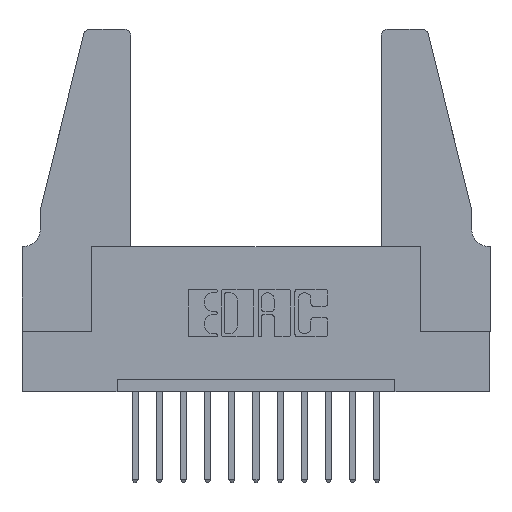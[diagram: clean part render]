
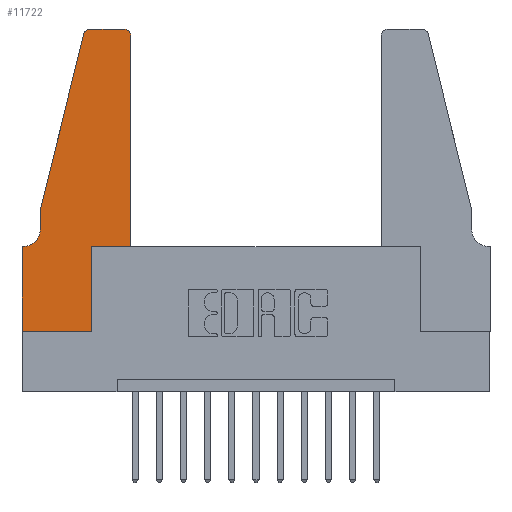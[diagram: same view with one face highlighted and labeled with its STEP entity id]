
A CAD part, top view. The second image highlights one B-rep face of the part: STEP entity #11722.
In plain terms, the highlighted planar face has unit normal (0, 0, 1).
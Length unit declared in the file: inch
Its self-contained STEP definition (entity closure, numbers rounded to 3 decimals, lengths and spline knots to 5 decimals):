
#106 = CARTESIAN_POINT ( 'NONE',  ( 0.2865, 0.35, 0.37 ) ) ;
#184 = VECTOR ( 'NONE', #12779, 39.37008 ) ;
#255 = DIRECTION ( 'NONE',  ( 1., 0., 0. ) ) ;
#328 = EDGE_CURVE ( 'NONE', #9432, #8564, #1690, .T. ) ;
#523 = EDGE_CURVE ( 'NONE', #2297, #10286, #2385, .T. ) ;
#626 = CARTESIAN_POINT ( 'NONE',  ( 0.2865, 0.35, 0.37 ) ) ;
#1080 = VECTOR ( 'NONE', #8777, 39.37008 ) ;
#1159 = VERTEX_POINT ( 'NONE', #5173 ) ;
#1486 = DIRECTION ( 'NONE',  ( 0., 1., 0. ) ) ;
#1690 = LINE ( 'NONE', #4432, #4351 ) ;
#1778 = DIRECTION ( 'NONE',  ( 0., 0., 1. ) ) ;
#2086 = FACE_OUTER_BOUND ( 'NONE', #7490, .T. ) ;
#2182 = AXIS2_PLACEMENT_3D ( 'NONE', #9927, #2772, #255 ) ;
#2297 = VERTEX_POINT ( 'NONE', #6164 ) ;
#2361 = DIRECTION ( 'NONE',  ( 1., 0., 0. ) ) ;
#2385 = LINE ( 'NONE', #5714, #5429 ) ;
#2461 = LINE ( 'NONE', #3813, #184 ) ;
#2501 = LINE ( 'NONE', #11528, #12940 ) ;
#2772 = DIRECTION ( 'NONE',  ( 0., 0., 1. ) ) ;
#2889 = EDGE_CURVE ( 'NONE', #3412, #6886, #9743, .T. ) ;
#2923 = PLANE ( 'NONE',  #6577 ) ;
#3412 = VERTEX_POINT ( 'NONE', #5383 ) ;
#3575 = DIRECTION ( 'NONE',  ( -1., 0., 0. ) ) ;
#3598 = VERTEX_POINT ( 'NONE', #626 ) ;
#3783 = ORIENTED_EDGE ( 'NONE', *, *, #9780, .T. ) ;
#3813 = CARTESIAN_POINT ( 'NONE',  ( 0., 0., 0.37 ) ) ;
#3838 = VERTEX_POINT ( 'NONE', #14155 ) ;
#4065 = VECTOR ( 'NONE', #5599, 39.37008 ) ;
#4280 = EDGE_CURVE ( 'NONE', #4663, #13851, #6752, .T. ) ;
#4351 = VECTOR ( 'NONE', #1486, 39.37008 ) ;
#4400 = ORIENTED_EDGE ( 'NONE', *, *, #328, .T. ) ;
#4432 = CARTESIAN_POINT ( 'NONE',  ( 0.4505, 0.35, 0.37 ) ) ;
#4453 = LINE ( 'NONE', #106, #7327 ) ;
#4565 = VECTOR ( 'NONE', #3575, 39.37008 ) ;
#4603 = CARTESIAN_POINT ( 'NONE',  ( 0.4205, 1.22, 0.37 ) ) ;
#4663 = VERTEX_POINT ( 'NONE', #6676 ) ;
#4938 = EDGE_CURVE ( 'NONE', #6886, #1159, #13020, .T. ) ;
#5011 = CARTESIAN_POINT ( 'NONE',  ( 0.0755, 0.35, 0.37 ) ) ;
#5173 = CARTESIAN_POINT ( 'NONE',  ( 0.25487, 1.22718, 0.37 ) ) ;
#5205 = CARTESIAN_POINT ( 'NONE',  ( 0.2865, 0., 0.37 ) ) ;
#5383 = CARTESIAN_POINT ( 'NONE',  ( 0.4205, 1.25, 0.37 ) ) ;
#5429 = VECTOR ( 'NONE', #11119, 39.37008 ) ;
#5599 = DIRECTION ( 'NONE',  ( 1., 0., 0. ) ) ;
#5714 = CARTESIAN_POINT ( 'NONE',  ( 0., 0., 0.37 ) ) ;
#5742 = LINE ( 'NONE', #10229, #7166 ) ;
#6142 = CARTESIAN_POINT ( 'NONE',  ( 0.0055, 0.42, 0.37 ) ) ;
#6164 = CARTESIAN_POINT ( 'NONE',  ( 0., 0., 0.37 ) ) ;
#6577 = AXIS2_PLACEMENT_3D ( 'NONE', #10827, #1778, #12131 ) ;
#6608 = ORIENTED_EDGE ( 'NONE', *, *, #12742, .T. ) ;
#6676 = CARTESIAN_POINT ( 'NONE',  ( 0.0055, 0.35, 0.37 ) ) ;
#6743 = ORIENTED_EDGE ( 'NONE', *, *, #4938, .T. ) ;
#6752 = LINE ( 'NONE', #5011, #4565 ) ;
#6780 = LINE ( 'NONE', #13635, #4065 ) ;
#6886 = VERTEX_POINT ( 'NONE', #11855 ) ;
#7166 = VECTOR ( 'NONE', #13763, 39.37008 ) ;
#7207 = EDGE_CURVE ( 'NONE', #1159, #8134, #2501, .T. ) ;
#7327 = VECTOR ( 'NONE', #9390, 39.37008 ) ;
#7490 = EDGE_LOOP ( 'NONE', ( #14387, #6743, #8351, #11825, #6608, #12822, #9866, #13274, #3783, #12224, #4400, #11113 ) ) ;
#8134 = VERTEX_POINT ( 'NONE', #13131 ) ;
#8351 = ORIENTED_EDGE ( 'NONE', *, *, #7207, .T. ) ;
#8386 = DIRECTION ( 'NONE',  ( -1., 0., 0. ) ) ;
#8564 = VERTEX_POINT ( 'NONE', #12717 ) ;
#8777 = DIRECTION ( 'NONE',  ( -1., 0., 0. ) ) ;
#9051 = EDGE_CURVE ( 'NONE', #8134, #3838, #5742, .T. ) ;
#9390 = DIRECTION ( 'NONE',  ( 0., 1., 0. ) ) ;
#9432 = VERTEX_POINT ( 'NONE', #13254 ) ;
#9743 = LINE ( 'NONE', #13363, #1080 ) ;
#9780 = EDGE_CURVE ( 'NONE', #10286, #3598, #4453, .T. ) ;
#9866 = ORIENTED_EDGE ( 'NONE', *, *, #10923, .T. ) ;
#9927 = CARTESIAN_POINT ( 'NONE',  ( 0.284, 1.22, 0.37 ) ) ;
#10229 = CARTESIAN_POINT ( 'NONE',  ( 0.0755, 0.5, 0.37 ) ) ;
#10286 = VERTEX_POINT ( 'NONE', #5205 ) ;
#10606 = EDGE_CURVE ( 'NONE', #3598, #9432, #6780, .T. ) ;
#10680 = AXIS2_PLACEMENT_3D ( 'NONE', #6142, #14030, #8386 ) ;
#10827 = CARTESIAN_POINT ( 'NONE',  ( 0., 0.35, 0.37 ) ) ;
#10923 = EDGE_CURVE ( 'NONE', #13851, #2297, #2461, .T. ) ;
#11113 = ORIENTED_EDGE ( 'NONE', *, *, #12006, .T. ) ;
#11119 = DIRECTION ( 'NONE',  ( 1., 0., 0. ) ) ;
#11528 = CARTESIAN_POINT ( 'NONE',  ( 0.0755, 0.5, 0.37 ) ) ;
#11542 = AXIS2_PLACEMENT_3D ( 'NONE', #4603, #12513, #2361 ) ;
#11722 = ADVANCED_FACE ( 'NONE', ( #2086 ), #2923, .T. ) ;
#11825 = ORIENTED_EDGE ( 'NONE', *, *, #9051, .T. ) ;
#11855 = CARTESIAN_POINT ( 'NONE',  ( 0.284, 1.25, 0.37 ) ) ;
#12006 = EDGE_CURVE ( 'NONE', #8564, #3412, #13942, .T. ) ;
#12131 = DIRECTION ( 'NONE',  ( 1., 0., 0. ) ) ;
#12142 = CIRCLE ( 'NONE', #10680, 0.07 ) ;
#12224 = ORIENTED_EDGE ( 'NONE', *, *, #10606, .T. ) ;
#12513 = DIRECTION ( 'NONE',  ( 0., 0., 1. ) ) ;
#12717 = CARTESIAN_POINT ( 'NONE',  ( 0.4505, 1.22, 0.37 ) ) ;
#12742 = EDGE_CURVE ( 'NONE', #3838, #4663, #12142, .T. ) ;
#12779 = DIRECTION ( 'NONE',  ( 0., -1., 0. ) ) ;
#12822 = ORIENTED_EDGE ( 'NONE', *, *, #4280, .T. ) ;
#12940 = VECTOR ( 'NONE', #13811, 39.37008 ) ;
#13020 = CIRCLE ( 'NONE', #2182, 0.03 ) ;
#13131 = CARTESIAN_POINT ( 'NONE',  ( 0.0755, 0.5, 0.37 ) ) ;
#13254 = CARTESIAN_POINT ( 'NONE',  ( 0.4505, 0.35, 0.37 ) ) ;
#13274 = ORIENTED_EDGE ( 'NONE', *, *, #523, .T. ) ;
#13363 = CARTESIAN_POINT ( 'NONE',  ( 0.2605, 1.25, 0.37 ) ) ;
#13635 = CARTESIAN_POINT ( 'NONE',  ( 0.4505, 0.35, 0.37 ) ) ;
#13763 = DIRECTION ( 'NONE',  ( 0., -1., 0. ) ) ;
#13811 = DIRECTION ( 'NONE',  ( -0.239, -0.971, 0. ) ) ;
#13851 = VERTEX_POINT ( 'NONE', #14476 ) ;
#13942 = CIRCLE ( 'NONE', #11542, 0.03 ) ;
#14030 = DIRECTION ( 'NONE',  ( 0., 0., -1. ) ) ;
#14155 = CARTESIAN_POINT ( 'NONE',  ( 0.0755, 0.42, 0.37 ) ) ;
#14387 = ORIENTED_EDGE ( 'NONE', *, *, #2889, .T. ) ;
#14476 = CARTESIAN_POINT ( 'NONE',  ( 0., 0.35, 0.37 ) ) ;
